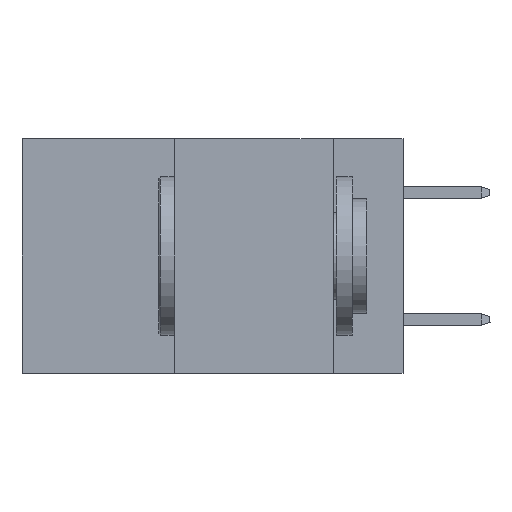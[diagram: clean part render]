
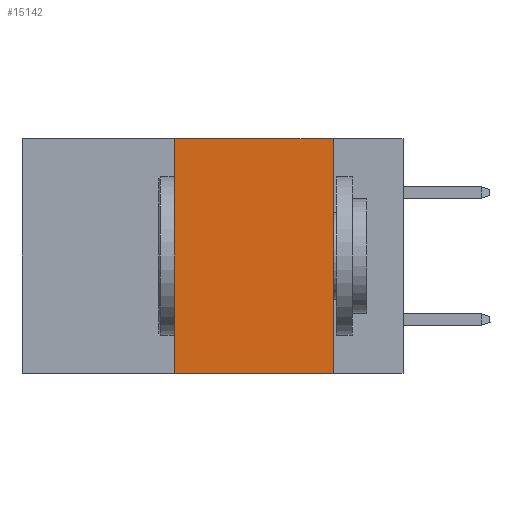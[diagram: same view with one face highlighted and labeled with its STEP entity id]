
A CAD part, left-side view. The second image highlights one B-rep face of the part: STEP entity #15142.
In plain terms, the highlighted planar face has unit normal (-1, 0, 0).
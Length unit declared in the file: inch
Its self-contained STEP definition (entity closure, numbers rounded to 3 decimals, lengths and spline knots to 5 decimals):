
#37 = CARTESIAN_POINT ( 'NONE',  ( 0., 0.6, 0. ) ) ;
#949 = VERTEX_POINT ( 'NONE', #11284 ) ;
#1876 = ORIENTED_EDGE ( 'NONE', *, *, #3279, .F. ) ;
#2064 = VERTEX_POINT ( 'NONE', #15905 ) ;
#2789 = DIRECTION ( 'NONE',  ( 0., 0., -1. ) ) ;
#3004 = DIRECTION ( 'NONE',  ( 0., 0., -1. ) ) ;
#3131 = EDGE_CURVE ( 'NONE', #8964, #2064, #11441, .T. ) ;
#3279 = EDGE_CURVE ( 'NONE', #949, #15244, #11808, .T. ) ;
#4465 = PLANE ( 'NONE',  #9726 ) ;
#4931 = EDGE_CURVE ( 'NONE', #8964, #949, #11063, .T. ) ;
#5212 = CARTESIAN_POINT ( 'NONE',  ( 0., 0.11, 0. ) ) ;
#5680 = DIRECTION ( 'NONE',  ( 1., 0., 0. ) ) ;
#5819 = DIRECTION ( 'NONE',  ( 0., -1., 0. ) ) ;
#8044 = VECTOR ( 'NONE', #5819, 39.37008 ) ;
#8285 = CARTESIAN_POINT ( 'NONE',  ( 0., 0.36, 0. ) ) ;
#8964 = VERTEX_POINT ( 'NONE', #13439 ) ;
#8980 = EDGE_CURVE ( 'NONE', #15244, #2064, #15069, .T. ) ;
#9044 = CARTESIAN_POINT ( 'NONE',  ( 0., 0.6, 0. ) ) ;
#9256 = VECTOR ( 'NONE', #9862, 39.37008 ) ;
#9289 = ORIENTED_EDGE ( 'NONE', *, *, #8980, .F. ) ;
#9726 = AXIS2_PLACEMENT_3D ( 'NONE', #37, #5680, #3004 ) ;
#9862 = DIRECTION ( 'NONE',  ( 0., 0., 1. ) ) ;
#10493 = VECTOR ( 'NONE', #2789, 39.37008 ) ;
#11063 = LINE ( 'NONE', #8285, #9256 ) ;
#11284 = CARTESIAN_POINT ( 'NONE',  ( 0., 0.36, 0. ) ) ;
#11441 = LINE ( 'NONE', #16891, #8044 ) ;
#11481 = FACE_OUTER_BOUND ( 'NONE', #12880, .T. ) ;
#11808 = LINE ( 'NONE', #9044, #11829 ) ;
#11829 = VECTOR ( 'NONE', #17160, 39.37008 ) ;
#12573 = CARTESIAN_POINT ( 'NONE',  ( 0., 0.11, 0. ) ) ;
#12880 = EDGE_LOOP ( 'NONE', ( #9289, #1876, #15317, #13241 ) ) ;
#13241 = ORIENTED_EDGE ( 'NONE', *, *, #3131, .T. ) ;
#13439 = CARTESIAN_POINT ( 'NONE',  ( 0., 0.36, -0.37 ) ) ;
#15069 = LINE ( 'NONE', #5212, #10493 ) ;
#15142 = ADVANCED_FACE ( 'NONE', ( #11481 ), #4465, .F. ) ;
#15244 = VERTEX_POINT ( 'NONE', #12573 ) ;
#15317 = ORIENTED_EDGE ( 'NONE', *, *, #4931, .F. ) ;
#15905 = CARTESIAN_POINT ( 'NONE',  ( 0., 0.11, -0.37 ) ) ;
#16891 = CARTESIAN_POINT ( 'NONE',  ( 0., 0.6, -0.37 ) ) ;
#17160 = DIRECTION ( 'NONE',  ( 0., -1., 0. ) ) ;
